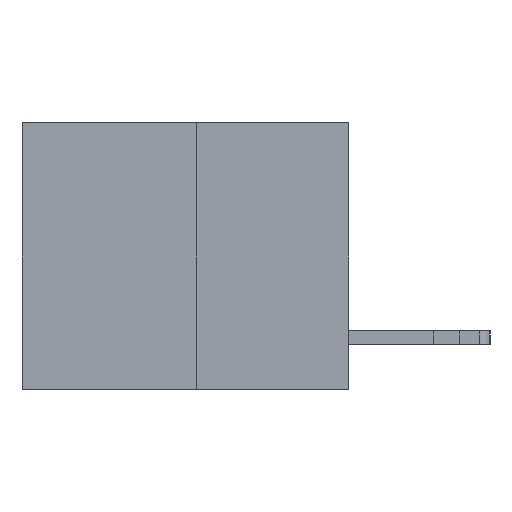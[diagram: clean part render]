
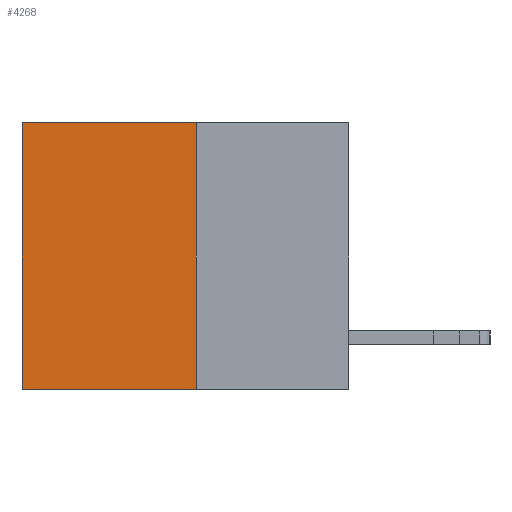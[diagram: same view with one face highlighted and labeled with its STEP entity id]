
A CAD part, left-side view. The second image highlights one B-rep face of the part: STEP entity #4268.
In plain terms, the highlighted planar face has unit normal (-1, 0, 0).
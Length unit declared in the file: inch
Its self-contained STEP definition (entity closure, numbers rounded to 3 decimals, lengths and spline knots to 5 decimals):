
#105 = DIRECTION ( 'NONE',  ( 1., 0., 0. ) ) ;
#886 = EDGE_CURVE ( 'NONE', #5604, #5893, #12648, .T. ) ;
#1100 = VECTOR ( 'NONE', #5922, 39.37008 ) ;
#1311 = ORIENTED_EDGE ( 'NONE', *, *, #11133, .T. ) ;
#1795 = LINE ( 'NONE', #6822, #1100 ) ;
#2334 = DIRECTION ( 'NONE',  ( 0., 0., -1. ) ) ;
#3178 = CARTESIAN_POINT ( 'NONE',  ( 0.3165, 0.28, 0. ) ) ;
#3184 = VERTEX_POINT ( 'NONE', #6882 ) ;
#4268 = ADVANCED_FACE ( 'NONE', ( #12363 ), #6666, .F. ) ;
#4649 = CARTESIAN_POINT ( 'NONE',  ( 0.3165, 0.28, 0. ) ) ;
#4752 = EDGE_CURVE ( 'NONE', #3184, #5893, #11440, .T. ) ;
#5075 = DIRECTION ( 'NONE',  ( 0., 1., 0. ) ) ;
#5340 = DIRECTION ( 'NONE',  ( 0., 1., 0. ) ) ;
#5604 = VERTEX_POINT ( 'NONE', #11619 ) ;
#5704 = ORIENTED_EDGE ( 'NONE', *, *, #11586, .F. ) ;
#5893 = VERTEX_POINT ( 'NONE', #9454 ) ;
#5922 = DIRECTION ( 'NONE',  ( 0., 0., -1. ) ) ;
#6192 = VECTOR ( 'NONE', #5340, 39.37008 ) ;
#6347 = LINE ( 'NONE', #3178, #6192 ) ;
#6561 = CARTESIAN_POINT ( 'NONE',  ( 0.3165, 0.28, -0.49 ) ) ;
#6594 = DIRECTION ( 'NONE',  ( 0., 0., -1. ) ) ;
#6666 = PLANE ( 'NONE',  #11667 ) ;
#6775 = EDGE_LOOP ( 'NONE', ( #7250, #9387, #5704, #1311 ) ) ;
#6822 = CARTESIAN_POINT ( 'NONE',  ( 0.3165, 0.28, -0.49 ) ) ;
#6882 = CARTESIAN_POINT ( 'NONE',  ( 0.3165, 0.28, -0.49 ) ) ;
#7250 = ORIENTED_EDGE ( 'NONE', *, *, #886, .T. ) ;
#8285 = CARTESIAN_POINT ( 'NONE',  ( 0.3165, 0.28, -0.49 ) ) ;
#8421 = VERTEX_POINT ( 'NONE', #4649 ) ;
#9387 = ORIENTED_EDGE ( 'NONE', *, *, #4752, .F. ) ;
#9454 = CARTESIAN_POINT ( 'NONE',  ( 0.3165, 0.6, -0.49 ) ) ;
#9789 = VECTOR ( 'NONE', #6594, 39.37008 ) ;
#9906 = CARTESIAN_POINT ( 'NONE',  ( 0.3165, 0.6, -0.49 ) ) ;
#11109 = VECTOR ( 'NONE', #5075, 39.37008 ) ;
#11133 = EDGE_CURVE ( 'NONE', #8421, #5604, #6347, .T. ) ;
#11440 = LINE ( 'NONE', #8285, #11109 ) ;
#11586 = EDGE_CURVE ( 'NONE', #8421, #3184, #1795, .T. ) ;
#11619 = CARTESIAN_POINT ( 'NONE',  ( 0.3165, 0.6, 0. ) ) ;
#11667 = AXIS2_PLACEMENT_3D ( 'NONE', #6561, #105, #2334 ) ;
#12363 = FACE_OUTER_BOUND ( 'NONE', #6775, .T. ) ;
#12648 = LINE ( 'NONE', #9906, #9789 ) ;
